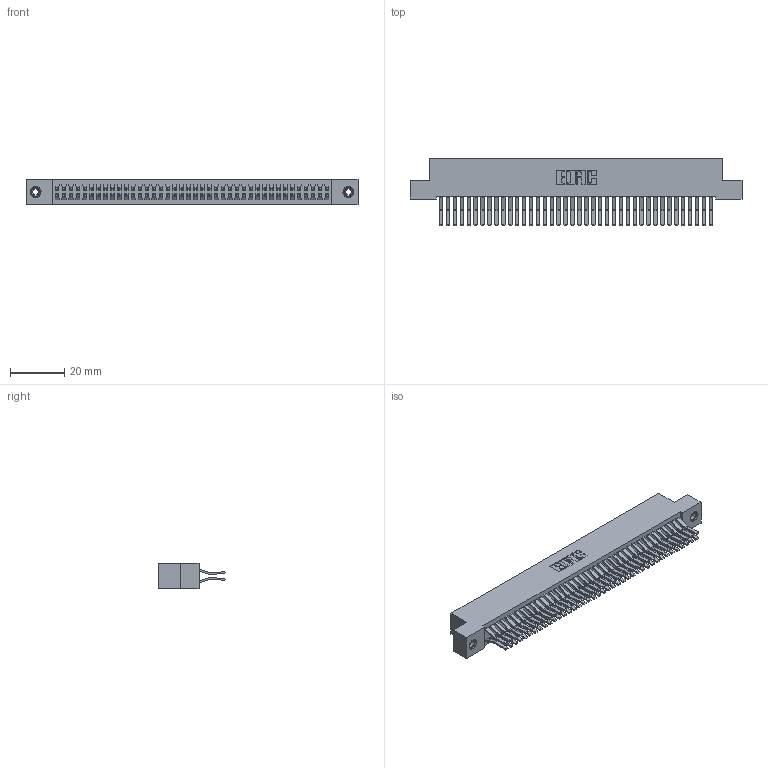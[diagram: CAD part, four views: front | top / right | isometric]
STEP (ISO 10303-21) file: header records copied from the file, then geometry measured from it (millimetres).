
FILE_DESCRIPTION (( 'STEP AP203' ), '1' );
FILE_NAME ('342-080-560-208.STEP', '2018-08-13T15:44:22', ( '' ), ( '' ), 'SwSTEP 2.0', 'SolidWorks 2016', '' );
FILE_SCHEMA (( 'CONFIG_CONTROL_DESIGN' ));
Length unit declared in the file: inch
Products named in the file (4): 345-250-001_345-250-003-102; 342 Part_TI; 342-080-560-208; 345-292-001_560 Tail
Assembly tree (83 placements, depth 2):
  342-080-560-208
    342 Part_TI
    345-292-001_560 Tail  x80
    345-250-001_345-250-003-102  x2
Bounding box: 121.92 x 24.78 x 9.4 mm (x, y, z)
Volume: 11464.6 mm3; surface area: 19881.9 mm2
Topology: 83 solids, 83 shells, 4490 faces, 13315 edges, 8762 vertices
Faces by surface type: plane 2978, cylinder 1496, cone 12, torus 4
Entity records: 27134 total; most frequent: CARTESIAN_POINT 4481, ORIENTED_EDGE 4410, DIRECTION 3867, EDGE_CURVE 2205, LINE 2053, VECTOR 2053, VERTEX_POINT 1464, AXIS2_PLACEMENT_3D 907
